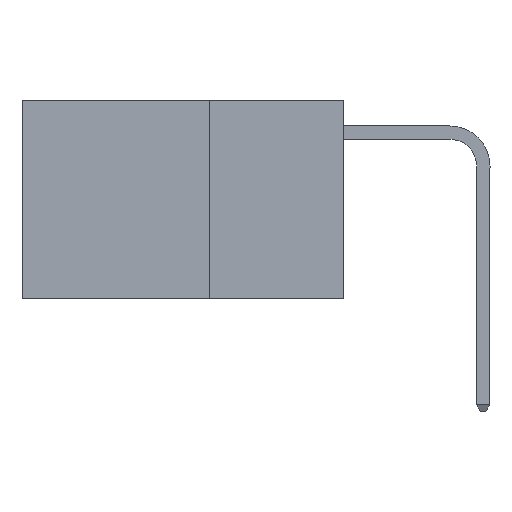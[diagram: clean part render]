
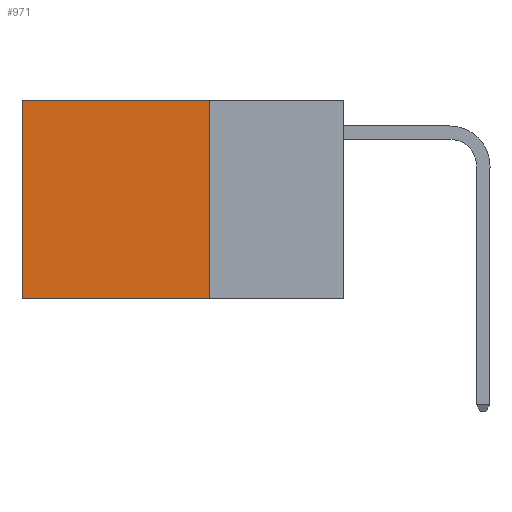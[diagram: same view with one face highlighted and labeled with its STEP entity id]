
A CAD part, left-side view. The second image highlights one B-rep face of the part: STEP entity #971.
In plain terms, the highlighted planar face has unit normal (-1, 0, 0).
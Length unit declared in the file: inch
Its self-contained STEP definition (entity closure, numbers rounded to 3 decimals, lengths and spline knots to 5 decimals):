
#315 = FACE_OUTER_BOUND ( 'NONE', #5928, .T. ) ;
#971 = ADVANCED_FACE ( 'NONE', ( #315 ), #5737, .F. ) ;
#1580 = AXIS2_PLACEMENT_3D ( 'NONE', #5682, #5577, #5255 ) ;
#2299 = LINE ( 'NONE', #6068, #2348 ) ;
#2348 = VECTOR ( 'NONE', #6545, 39.37008 ) ;
#2803 = CARTESIAN_POINT ( 'NONE',  ( 0.2625, 0.6, 0. ) ) ;
#2914 = EDGE_CURVE ( 'NONE', #5540, #11779, #2299, .T. ) ;
#3255 = CARTESIAN_POINT ( 'NONE',  ( 0.2625, 0.25, -0.37 ) ) ;
#3393 = CARTESIAN_POINT ( 'NONE',  ( 0.2625, 0.25, -0.37 ) ) ;
#3904 = ORIENTED_EDGE ( 'NONE', *, *, #8587, .T. ) ;
#4239 = VECTOR ( 'NONE', #4503, 39.37008 ) ;
#4254 = ORIENTED_EDGE ( 'NONE', *, *, #12861, .F. ) ;
#4372 = ORIENTED_EDGE ( 'NONE', *, *, #9546, .F. ) ;
#4437 = LINE ( 'NONE', #5325, #4239 ) ;
#4503 = DIRECTION ( 'NONE',  ( 0., 0., -1. ) ) ;
#4522 = ORIENTED_EDGE ( 'NONE', *, *, #2914, .T. ) ;
#5095 = CARTESIAN_POINT ( 'NONE',  ( 0.2625, 0.25, 0. ) ) ;
#5255 = DIRECTION ( 'NONE',  ( 0., 0., -1. ) ) ;
#5325 = CARTESIAN_POINT ( 'NONE',  ( 0.2625, 0.25, 0. ) ) ;
#5540 = VERTEX_POINT ( 'NONE', #5095 ) ;
#5577 = DIRECTION ( 'NONE',  ( 1., 0., 0. ) ) ;
#5659 = VERTEX_POINT ( 'NONE', #3255 ) ;
#5682 = CARTESIAN_POINT ( 'NONE',  ( 0.2625, 0.25, 0. ) ) ;
#5737 = PLANE ( 'NONE',  #1580 ) ;
#5928 = EDGE_LOOP ( 'NONE', ( #3904, #4254, #4372, #4522 ) ) ;
#6068 = CARTESIAN_POINT ( 'NONE',  ( 0.2625, 0.25, 0. ) ) ;
#6545 = DIRECTION ( 'NONE',  ( 0., 1., 0. ) ) ;
#8587 = EDGE_CURVE ( 'NONE', #11779, #12479, #13194, .T. ) ;
#9546 = EDGE_CURVE ( 'NONE', #5540, #5659, #4437, .T. ) ;
#11375 = CARTESIAN_POINT ( 'NONE',  ( 0.2625, 0.6, -0.37 ) ) ;
#11779 = VERTEX_POINT ( 'NONE', #2803 ) ;
#11918 = DIRECTION ( 'NONE',  ( 0., 1., 0. ) ) ;
#12372 = LINE ( 'NONE', #3393, #12383 ) ;
#12383 = VECTOR ( 'NONE', #11918, 39.37008 ) ;
#12479 = VERTEX_POINT ( 'NONE', #11375 ) ;
#12861 = EDGE_CURVE ( 'NONE', #5659, #12479, #12372, .T. ) ;
#12982 = CARTESIAN_POINT ( 'NONE',  ( 0.2625, 0.6, 0. ) ) ;
#13039 = VECTOR ( 'NONE', #13300, 39.37008 ) ;
#13194 = LINE ( 'NONE', #12982, #13039 ) ;
#13300 = DIRECTION ( 'NONE',  ( 0., 0., -1. ) ) ;
